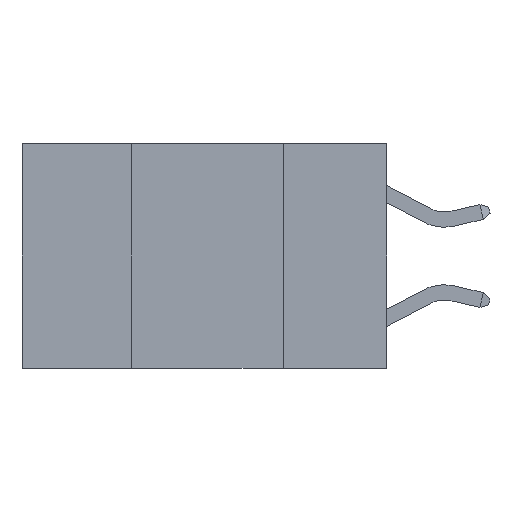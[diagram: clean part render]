
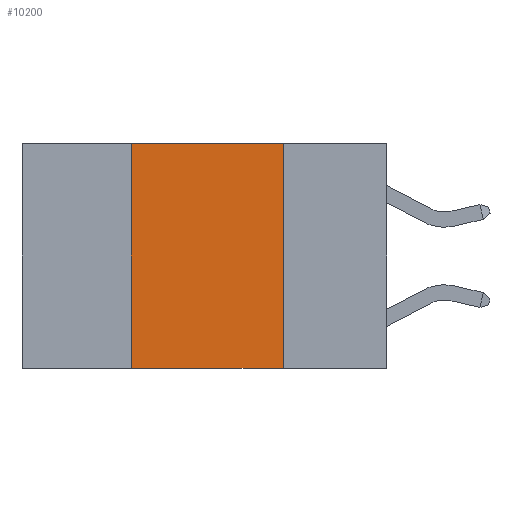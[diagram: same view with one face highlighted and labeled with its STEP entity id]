
A CAD part, left-side view. The second image highlights one B-rep face of the part: STEP entity #10200.
In plain terms, the highlighted planar face has unit normal (-1, 0, 0).
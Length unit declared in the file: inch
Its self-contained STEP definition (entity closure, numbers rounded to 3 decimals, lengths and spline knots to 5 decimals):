
#64 = EDGE_CURVE ( 'NONE', #3797, #4797, #6836, .T. ) ;
#65 = VECTOR ( 'NONE', #19182, 39.37008 ) ;
#143 = DIRECTION ( 'NONE',  ( 0., 0., -1. ) ) ;
#575 = LINE ( 'NONE', #6198, #65 ) ;
#1086 = DIRECTION ( 'NONE',  ( 0., 0., 1. ) ) ;
#1118 = VERTEX_POINT ( 'NONE', #14285 ) ;
#1358 = DIRECTION ( 'NONE',  ( 1., 0., 0. ) ) ;
#2215 = CARTESIAN_POINT ( 'NONE',  ( 0., 0.6, -0.37 ) ) ;
#2336 = EDGE_CURVE ( 'NONE', #1118, #14298, #8291, .T. ) ;
#3131 = PLANE ( 'NONE',  #14710 ) ;
#3797 = VERTEX_POINT ( 'NONE', #14249 ) ;
#3870 = CARTESIAN_POINT ( 'NONE',  ( 0., 0.17, -0.37 ) ) ;
#4797 = VERTEX_POINT ( 'NONE', #3870 ) ;
#4883 = VECTOR ( 'NONE', #13662, 39.37008 ) ;
#6198 = CARTESIAN_POINT ( 'NONE',  ( 0., 0.6, 0. ) ) ;
#6385 = CARTESIAN_POINT ( 'NONE',  ( 0., 0.6, 0. ) ) ;
#6459 = DIRECTION ( 'NONE',  ( 0., 0., -1. ) ) ;
#6836 = LINE ( 'NONE', #14960, #14971 ) ;
#8291 = LINE ( 'NONE', #9369, #20683 ) ;
#9369 = CARTESIAN_POINT ( 'NONE',  ( 0., 0.42, 0. ) ) ;
#10200 = ADVANCED_FACE ( 'NONE', ( #16279 ), #3131, .F. ) ;
#11358 = EDGE_CURVE ( 'NONE', #14298, #3797, #575, .T. ) ;
#13662 = DIRECTION ( 'NONE',  ( 0., -1., 0. ) ) ;
#14249 = CARTESIAN_POINT ( 'NONE',  ( 0., 0.17, 0. ) ) ;
#14285 = CARTESIAN_POINT ( 'NONE',  ( 0., 0.42, -0.37 ) ) ;
#14298 = VERTEX_POINT ( 'NONE', #17903 ) ;
#14520 = EDGE_CURVE ( 'NONE', #1118, #4797, #17305, .T. ) ;
#14710 = AXIS2_PLACEMENT_3D ( 'NONE', #6385, #1358, #6459 ) ;
#14960 = CARTESIAN_POINT ( 'NONE',  ( 0., 0.17, 0. ) ) ;
#14971 = VECTOR ( 'NONE', #143, 39.37008 ) ;
#15501 = EDGE_LOOP ( 'NONE', ( #18219, #19085, #18430, #18174 ) ) ;
#16279 = FACE_OUTER_BOUND ( 'NONE', #15501, .T. ) ;
#17305 = LINE ( 'NONE', #2215, #4883 ) ;
#17903 = CARTESIAN_POINT ( 'NONE',  ( 0., 0.42, 0. ) ) ;
#18174 = ORIENTED_EDGE ( 'NONE', *, *, #14520, .T. ) ;
#18219 = ORIENTED_EDGE ( 'NONE', *, *, #64, .F. ) ;
#18430 = ORIENTED_EDGE ( 'NONE', *, *, #2336, .F. ) ;
#19085 = ORIENTED_EDGE ( 'NONE', *, *, #11358, .F. ) ;
#19182 = DIRECTION ( 'NONE',  ( 0., -1., 0. ) ) ;
#20683 = VECTOR ( 'NONE', #1086, 39.37008 ) ;
